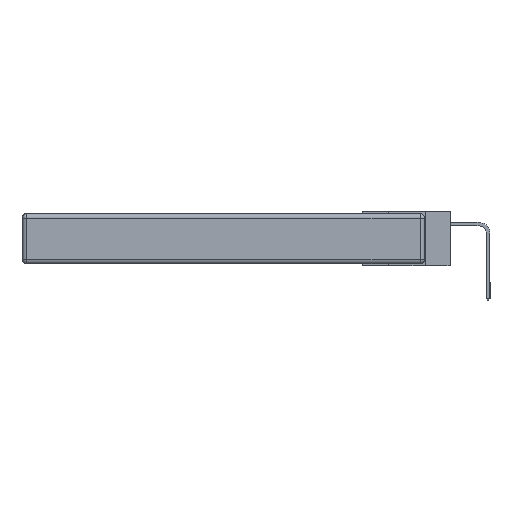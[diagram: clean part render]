
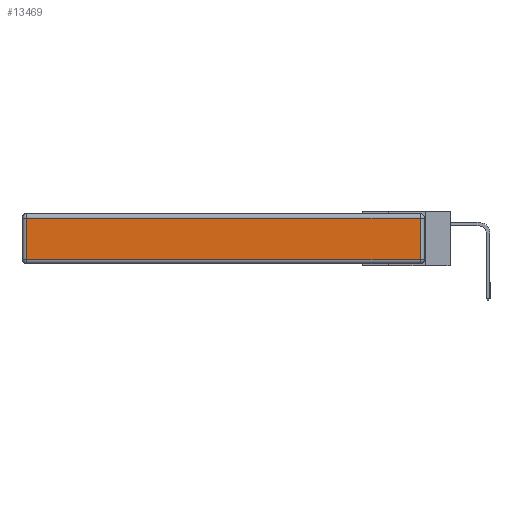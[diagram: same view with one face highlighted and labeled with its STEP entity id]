
A CAD part, left-side view. The second image highlights one B-rep face of the part: STEP entity #13469.
In plain terms, the highlighted planar face has unit normal (-1, 0, 0).
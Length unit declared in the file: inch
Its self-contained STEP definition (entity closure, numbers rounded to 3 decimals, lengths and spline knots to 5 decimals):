
#201 = DIRECTION ( 'NONE',  ( 0., 0., 1. ) ) ;
#644 = CARTESIAN_POINT ( 'NONE',  ( 0., 2.72, -0.03 ) ) ;
#1569 = DIRECTION ( 'NONE',  ( 0., 0., 1. ) ) ;
#1666 = PLANE ( 'NONE',  #9406 ) ;
#1986 = LINE ( 'NONE', #18905, #3958 ) ;
#2269 = VERTEX_POINT ( 'NONE', #10715 ) ;
#3958 = VECTOR ( 'NONE', #12798, 39.37008 ) ;
#4133 = EDGE_CURVE ( 'NONE', #16958, #7205, #12819, .T. ) ;
#6250 = VERTEX_POINT ( 'NONE', #14487 ) ;
#7200 = ORIENTED_EDGE ( 'NONE', *, *, #25405, .T. ) ;
#7205 = VERTEX_POINT ( 'NONE', #644 ) ;
#7640 = CARTESIAN_POINT ( 'NONE',  ( 0., 0.03, -0.03 ) ) ;
#9031 = ORIENTED_EDGE ( 'NONE', *, *, #4133, .T. ) ;
#9406 = AXIS2_PLACEMENT_3D ( 'NONE', #27008, #20761, #1569 ) ;
#9587 = CARTESIAN_POINT ( 'NONE',  ( 0., 0., -0.313 ) ) ;
#10715 = CARTESIAN_POINT ( 'NONE',  ( 0., 0.03, -0.313 ) ) ;
#11015 = CARTESIAN_POINT ( 'NONE',  ( 0., 0.03, -0.343 ) ) ;
#12798 = DIRECTION ( 'NONE',  ( 0., 0., -1. ) ) ;
#12819 = LINE ( 'NONE', #21272, #15475 ) ;
#13198 = EDGE_CURVE ( 'NONE', #6250, #2269, #19872, .T. ) ;
#13469 = ADVANCED_FACE ( 'NONE', ( #14849 ), #1666, .T. ) ;
#14233 = VECTOR ( 'NONE', #201, 39.37008 ) ;
#14487 = CARTESIAN_POINT ( 'NONE',  ( 0., 2.72, -0.313 ) ) ;
#14849 = FACE_OUTER_BOUND ( 'NONE', #16721, .T. ) ;
#15475 = VECTOR ( 'NONE', #23543, 39.37008 ) ;
#16721 = EDGE_LOOP ( 'NONE', ( #20646, #17089, #9031, #7200 ) ) ;
#16958 = VERTEX_POINT ( 'NONE', #7640 ) ;
#17089 = ORIENTED_EDGE ( 'NONE', *, *, #26140, .T. ) ;
#18905 = CARTESIAN_POINT ( 'NONE',  ( 0., 2.72, -0.343 ) ) ;
#19872 = LINE ( 'NONE', #9587, #22172 ) ;
#20222 = DIRECTION ( 'NONE',  ( 0., -1., 0. ) ) ;
#20646 = ORIENTED_EDGE ( 'NONE', *, *, #13198, .T. ) ;
#20761 = DIRECTION ( 'NONE',  ( -1., 0., 0. ) ) ;
#21272 = CARTESIAN_POINT ( 'NONE',  ( 0., 2.75, -0.03 ) ) ;
#22163 = LINE ( 'NONE', #11015, #14233 ) ;
#22172 = VECTOR ( 'NONE', #20222, 39.37008 ) ;
#23543 = DIRECTION ( 'NONE',  ( 0., 1., 0. ) ) ;
#25405 = EDGE_CURVE ( 'NONE', #7205, #6250, #1986, .T. ) ;
#26140 = EDGE_CURVE ( 'NONE', #2269, #16958, #22163, .T. ) ;
#27008 = CARTESIAN_POINT ( 'NONE',  ( 0., 0., -0.343 ) ) ;
